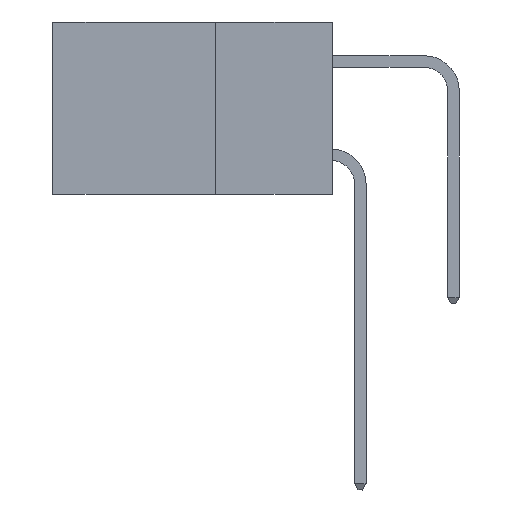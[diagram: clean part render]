
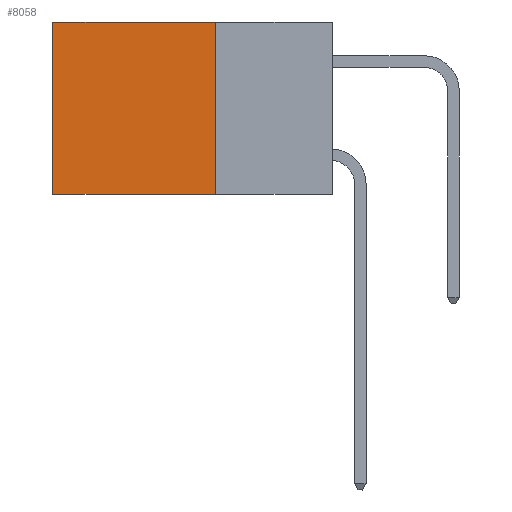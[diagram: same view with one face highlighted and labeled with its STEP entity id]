
A CAD part, left-side view. The second image highlights one B-rep face of the part: STEP entity #8058.
In plain terms, the highlighted planar face has unit normal (-1, 0, 0).
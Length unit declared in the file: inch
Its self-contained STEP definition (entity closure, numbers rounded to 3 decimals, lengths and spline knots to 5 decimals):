
#215 = VERTEX_POINT ( 'NONE', #14526 ) ;
#288 = EDGE_CURVE ( 'NONE', #11062, #215, #19669, .T. ) ;
#756 = DIRECTION ( 'NONE',  ( 1., 0., 0. ) ) ;
#2216 = ORIENTED_EDGE ( 'NONE', *, *, #288, .T. ) ;
#2519 = CARTESIAN_POINT ( 'NONE',  ( 0.2615, 0.25, 0. ) ) ;
#3781 = CARTESIAN_POINT ( 'NONE',  ( 0.2615, 0.6, -0.37 ) ) ;
#3880 = FACE_OUTER_BOUND ( 'NONE', #14571, .T. ) ;
#5549 = DIRECTION ( 'NONE',  ( 0., 0., -1. ) ) ;
#6257 = ORIENTED_EDGE ( 'NONE', *, *, #6629, .F. ) ;
#6629 = EDGE_CURVE ( 'NONE', #7249, #10707, #19248, .T. ) ;
#6762 = EDGE_CURVE ( 'NONE', #10707, #215, #6910, .T. ) ;
#6910 = LINE ( 'NONE', #19660, #12810 ) ;
#6912 = PLANE ( 'NONE',  #14832 ) ;
#6977 = CARTESIAN_POINT ( 'NONE',  ( 0.2615, 0.6, 0. ) ) ;
#7015 = CARTESIAN_POINT ( 'NONE',  ( 0.2615, 0.25, -0.37 ) ) ;
#7249 = VERTEX_POINT ( 'NONE', #12319 ) ;
#7478 = ORIENTED_EDGE ( 'NONE', *, *, #19757, .T. ) ;
#8058 = ADVANCED_FACE ( 'NONE', ( #3880 ), #6912, .F. ) ;
#9795 = VECTOR ( 'NONE', #12971, 39.37008 ) ;
#10119 = DIRECTION ( 'NONE',  ( 0., 1., 0. ) ) ;
#10707 = VERTEX_POINT ( 'NONE', #19953 ) ;
#11062 = VERTEX_POINT ( 'NONE', #6977 ) ;
#11711 = DIRECTION ( 'NONE',  ( 0., 1., 0. ) ) ;
#12319 = CARTESIAN_POINT ( 'NONE',  ( 0.2615, 0.25, 0. ) ) ;
#12810 = VECTOR ( 'NONE', #11711, 39.37008 ) ;
#12971 = DIRECTION ( 'NONE',  ( 0., 0., -1. ) ) ;
#13573 = ORIENTED_EDGE ( 'NONE', *, *, #6762, .F. ) ;
#14123 = DIRECTION ( 'NONE',  ( 0., 0., -1. ) ) ;
#14526 = CARTESIAN_POINT ( 'NONE',  ( 0.2615, 0.6, -0.37 ) ) ;
#14571 = EDGE_LOOP ( 'NONE', ( #2216, #13573, #6257, #7478 ) ) ;
#14832 = AXIS2_PLACEMENT_3D ( 'NONE', #7015, #756, #5549 ) ;
#15801 = CARTESIAN_POINT ( 'NONE',  ( 0.2615, 0.25, -0.37 ) ) ;
#16558 = VECTOR ( 'NONE', #10119, 39.37008 ) ;
#18167 = VECTOR ( 'NONE', #14123, 39.37008 ) ;
#18296 = LINE ( 'NONE', #2519, #16558 ) ;
#19248 = LINE ( 'NONE', #15801, #18167 ) ;
#19660 = CARTESIAN_POINT ( 'NONE',  ( 0.2615, 0.25, -0.37 ) ) ;
#19669 = LINE ( 'NONE', #3781, #9795 ) ;
#19757 = EDGE_CURVE ( 'NONE', #7249, #11062, #18296, .T. ) ;
#19953 = CARTESIAN_POINT ( 'NONE',  ( 0.2615, 0.25, -0.37 ) ) ;
